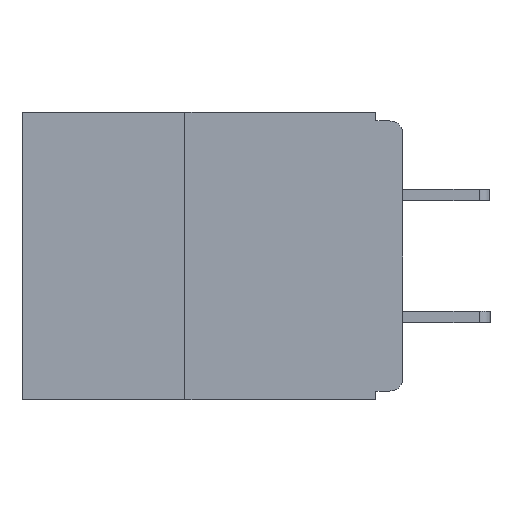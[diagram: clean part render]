
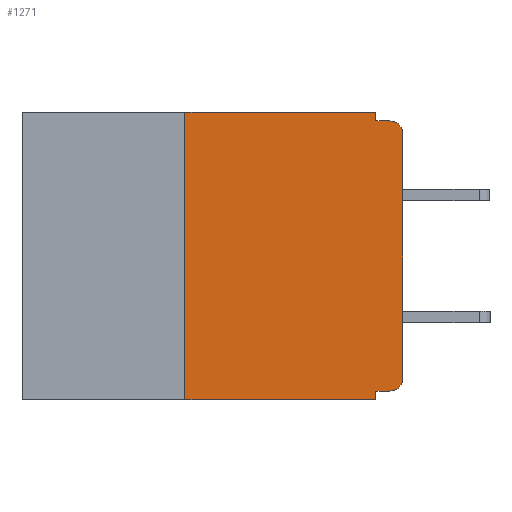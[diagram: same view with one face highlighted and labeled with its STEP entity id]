
A CAD part, left-side view. The second image highlights one B-rep face of the part: STEP entity #1271.
In plain terms, the highlighted planar face has unit normal (-1, 0, 0).
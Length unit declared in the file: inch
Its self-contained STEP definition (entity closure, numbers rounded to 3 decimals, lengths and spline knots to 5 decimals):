
#10 = VERTEX_POINT ( 'NONE', #12020 ) ;
#320 = PLANE ( 'NONE',  #678 ) ;
#678 = AXIS2_PLACEMENT_3D ( 'NONE', #16338, #2193, #15969 ) ;
#800 = EDGE_CURVE ( 'NONE', #4495, #4245, #7975, .T. ) ;
#861 = VECTOR ( 'NONE', #13200, 39.37008 ) ;
#929 = CARTESIAN_POINT ( 'NONE',  ( 0., 0., 0. ) ) ;
#1073 = CARTESIAN_POINT ( 'NONE',  ( 0., 0.25, -0.33 ) ) ;
#1226 = EDGE_CURVE ( 'NONE', #14212, #13061, #8919, .T. ) ;
#1271 = ADVANCED_FACE ( 'NONE', ( #1846 ), #320, .F. ) ;
#1317 = VECTOR ( 'NONE', #6708, 39.37008 ) ;
#1846 = FACE_OUTER_BOUND ( 'NONE', #4901, .T. ) ;
#2112 = EDGE_CURVE ( 'NONE', #14538, #4964, #9324, .T. ) ;
#2193 = DIRECTION ( 'NONE',  ( 1., 0., 0. ) ) ;
#2389 = DIRECTION ( 'NONE',  ( 0., 0., -1. ) ) ;
#2770 = CARTESIAN_POINT ( 'NONE',  ( 0., 0.031, -0.01 ) ) ;
#2789 = DIRECTION ( 'NONE',  ( 0., -1., 0. ) ) ;
#3219 = CIRCLE ( 'NONE', #7208, 0.015 ) ;
#3656 = ORIENTED_EDGE ( 'NONE', *, *, #6363, .F. ) ;
#4245 = VERTEX_POINT ( 'NONE', #2770 ) ;
#4310 = VERTEX_POINT ( 'NONE', #19209 ) ;
#4495 = VERTEX_POINT ( 'NONE', #15919 ) ;
#4769 = EDGE_CURVE ( 'NONE', #4245, #4310, #9013, .T. ) ;
#4901 = EDGE_LOOP ( 'NONE', ( #8945, #16095, #6776, #15896, #3656, #14540, #7237, #11221, #12153, #5824 ) ) ;
#4964 = VERTEX_POINT ( 'NONE', #7926 ) ;
#5126 = CARTESIAN_POINT ( 'NONE',  ( 0., 0.031, 0. ) ) ;
#5313 = CARTESIAN_POINT ( 'NONE',  ( 0., 0.015, -0.305 ) ) ;
#5424 = DIRECTION ( 'NONE',  ( -1., 0., 0. ) ) ;
#5541 = CARTESIAN_POINT ( 'NONE',  ( 0., 0.031, -0.32 ) ) ;
#5557 = CARTESIAN_POINT ( 'NONE',  ( 0., 0.25, -0.33 ) ) ;
#5824 = ORIENTED_EDGE ( 'NONE', *, *, #13606, .T. ) ;
#6363 = EDGE_CURVE ( 'NONE', #4964, #4495, #19336, .T. ) ;
#6708 = DIRECTION ( 'NONE',  ( 0., 0., 1. ) ) ;
#6728 = AXIS2_PLACEMENT_3D ( 'NONE', #14570, #5424, #16062 ) ;
#6776 = ORIENTED_EDGE ( 'NONE', *, *, #4769, .F. ) ;
#6864 = DIRECTION ( 'NONE',  ( 0., 0., -1. ) ) ;
#7021 = VECTOR ( 'NONE', #19052, 39.37008 ) ;
#7208 = AXIS2_PLACEMENT_3D ( 'NONE', #5313, #15952, #6864 ) ;
#7237 = ORIENTED_EDGE ( 'NONE', *, *, #10287, .T. ) ;
#7513 = LINE ( 'NONE', #929, #7021 ) ;
#7926 = CARTESIAN_POINT ( 'NONE',  ( 0., 0.25, 0. ) ) ;
#7975 = LINE ( 'NONE', #5126, #19561 ) ;
#8919 = LINE ( 'NONE', #13317, #861 ) ;
#8945 = ORIENTED_EDGE ( 'NONE', *, *, #18476, .T. ) ;
#9013 = LINE ( 'NONE', #11809, #16627 ) ;
#9200 = EDGE_CURVE ( 'NONE', #12019, #4310, #13329, .T. ) ;
#9324 = LINE ( 'NONE', #5557, #1317 ) ;
#9397 = VECTOR ( 'NONE', #17450, 39.37008 ) ;
#9800 = CARTESIAN_POINT ( 'NONE',  ( 0., 0.437, -0.33 ) ) ;
#9864 = LINE ( 'NONE', #9800, #9397 ) ;
#9975 = CARTESIAN_POINT ( 'NONE',  ( 0., 0., -0.305 ) ) ;
#10287 = EDGE_CURVE ( 'NONE', #14538, #10, #9864, .T. ) ;
#11017 = VERTEX_POINT ( 'NONE', #9975 ) ;
#11221 = ORIENTED_EDGE ( 'NONE', *, *, #17584, .F. ) ;
#11310 = VECTOR ( 'NONE', #2789, 39.37008 ) ;
#11543 = DIRECTION ( 'NONE',  ( 0., -1., 0. ) ) ;
#11809 = CARTESIAN_POINT ( 'NONE',  ( 0., 0., -0.01 ) ) ;
#11821 = CARTESIAN_POINT ( 'NONE',  ( 0., 0.437, 0. ) ) ;
#12019 = VERTEX_POINT ( 'NONE', #13607 ) ;
#12020 = CARTESIAN_POINT ( 'NONE',  ( 0., 0.031, -0.33 ) ) ;
#12153 = ORIENTED_EDGE ( 'NONE', *, *, #1226, .F. ) ;
#12168 = DIRECTION ( 'NONE',  ( 0., 0., -1. ) ) ;
#13061 = VERTEX_POINT ( 'NONE', #5541 ) ;
#13200 = DIRECTION ( 'NONE',  ( 0., 1., 0. ) ) ;
#13317 = CARTESIAN_POINT ( 'NONE',  ( 0., 0., -0.32 ) ) ;
#13329 = CIRCLE ( 'NONE', #6728, 0.015 ) ;
#13606 = EDGE_CURVE ( 'NONE', #14212, #11017, #3219, .T. ) ;
#13607 = CARTESIAN_POINT ( 'NONE',  ( 0., 0., -0.025 ) ) ;
#13988 = CARTESIAN_POINT ( 'NONE',  ( 0., 0.015, -0.32 ) ) ;
#14212 = VERTEX_POINT ( 'NONE', #13988 ) ;
#14538 = VERTEX_POINT ( 'NONE', #1073 ) ;
#14540 = ORIENTED_EDGE ( 'NONE', *, *, #2112, .F. ) ;
#14570 = CARTESIAN_POINT ( 'NONE',  ( 0., 0.015, -0.025 ) ) ;
#15623 = VECTOR ( 'NONE', #12168, 39.37008 ) ;
#15896 = ORIENTED_EDGE ( 'NONE', *, *, #800, .F. ) ;
#15919 = CARTESIAN_POINT ( 'NONE',  ( 0., 0.031, 0. ) ) ;
#15952 = DIRECTION ( 'NONE',  ( -1., 0., 0. ) ) ;
#15969 = DIRECTION ( 'NONE',  ( 0., 0., -1. ) ) ;
#16062 = DIRECTION ( 'NONE',  ( 0., 0., -1. ) ) ;
#16095 = ORIENTED_EDGE ( 'NONE', *, *, #9200, .T. ) ;
#16338 = CARTESIAN_POINT ( 'NONE',  ( 0., 0.437, 0. ) ) ;
#16627 = VECTOR ( 'NONE', #11543, 39.37008 ) ;
#17450 = DIRECTION ( 'NONE',  ( 0., -1., 0. ) ) ;
#17584 = EDGE_CURVE ( 'NONE', #13061, #10, #19577, .T. ) ;
#18207 = CARTESIAN_POINT ( 'NONE',  ( 0., 0.031, -0.33 ) ) ;
#18476 = EDGE_CURVE ( 'NONE', #11017, #12019, #7513, .T. ) ;
#19052 = DIRECTION ( 'NONE',  ( 0., 0., 1. ) ) ;
#19209 = CARTESIAN_POINT ( 'NONE',  ( 0., 0.015, -0.01 ) ) ;
#19336 = LINE ( 'NONE', #11821, #11310 ) ;
#19561 = VECTOR ( 'NONE', #2389, 39.37008 ) ;
#19577 = LINE ( 'NONE', #18207, #15623 ) ;
